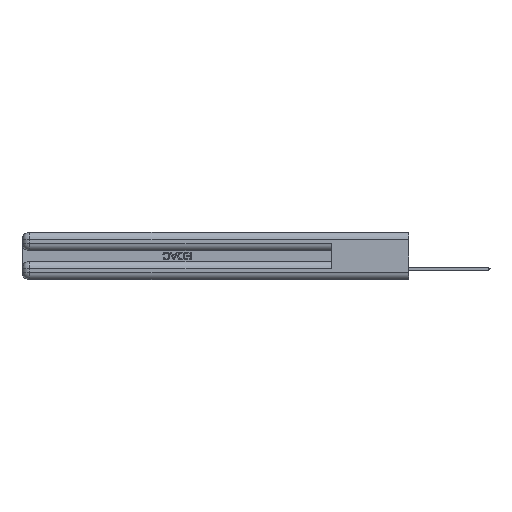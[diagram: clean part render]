
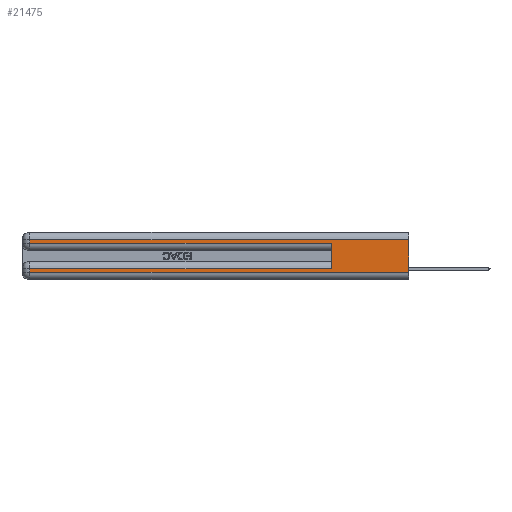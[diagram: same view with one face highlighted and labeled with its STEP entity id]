
A CAD part, left-side view. The second image highlights one B-rep face of the part: STEP entity #21475.
In plain terms, the highlighted planar face has unit normal (-1, 0, 0).
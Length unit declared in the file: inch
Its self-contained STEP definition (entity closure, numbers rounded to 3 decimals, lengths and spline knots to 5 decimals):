
#2013 = VECTOR ( 'NONE', #28800, 39.37008 ) ;
#2244 = DIRECTION ( 'NONE',  ( 0., 0., -1. ) ) ;
#2348 = AXIS2_PLACEMENT_3D ( 'NONE', #2949, #3108, #23574 ) ;
#2818 = DIRECTION ( 'NONE',  ( 0., -1., 0. ) ) ;
#2949 = CARTESIAN_POINT ( 'NONE',  ( 0., 0., 0.37 ) ) ;
#3108 = DIRECTION ( 'NONE',  ( 1., 0., 0. ) ) ;
#3321 = EDGE_CURVE ( 'NONE', #38201, #8779, #11800, .T. ) ;
#3436 = LINE ( 'NONE', #38410, #30275 ) ;
#3728 = LINE ( 'NONE', #9782, #32764 ) ;
#5554 = VERTEX_POINT ( 'NONE', #9610 ) ;
#7257 = EDGE_CURVE ( 'NONE', #16103, #8779, #3728, .T. ) ;
#7358 = CARTESIAN_POINT ( 'NONE',  ( 0., 0., 0.31 ) ) ;
#8779 = VERTEX_POINT ( 'NONE', #22190 ) ;
#9610 = CARTESIAN_POINT ( 'NONE',  ( 0., 2.94, 0.085 ) ) ;
#9782 = CARTESIAN_POINT ( 'NONE',  ( 0., 0., 0.37 ) ) ;
#10537 = ORIENTED_EDGE ( 'NONE', *, *, #3321, .T. ) ;
#11504 = DIRECTION ( 'NONE',  ( 0., 0., -1. ) ) ;
#11552 = LINE ( 'NONE', #16297, #13139 ) ;
#11800 = LINE ( 'NONE', #13578, #14001 ) ;
#12268 = EDGE_CURVE ( 'NONE', #43119, #5554, #11552, .T. ) ;
#12500 = EDGE_LOOP ( 'NONE', ( #44395, #36918, #36871, #23551, #28373, #17682, #26992, #10537 ) ) ;
#13139 = VECTOR ( 'NONE', #19790, 39.37008 ) ;
#13212 = CARTESIAN_POINT ( 'NONE',  ( 0., 0.6, 0.285 ) ) ;
#13380 = VECTOR ( 'NONE', #19745, 39.37008 ) ;
#13578 = CARTESIAN_POINT ( 'NONE',  ( 0., 0., 0.06 ) ) ;
#13644 = CARTESIAN_POINT ( 'NONE',  ( 0., 0.6, 0.085 ) ) ;
#14001 = VECTOR ( 'NONE', #2818, 39.37008 ) ;
#16103 = VERTEX_POINT ( 'NONE', #7358 ) ;
#16235 = EDGE_CURVE ( 'NONE', #45149, #21847, #43623, .T. ) ;
#16279 = VECTOR ( 'NONE', #11504, 39.37008 ) ;
#16297 = CARTESIAN_POINT ( 'NONE',  ( 0., 0., 0.085 ) ) ;
#17682 = ORIENTED_EDGE ( 'NONE', *, *, #12268, .T. ) ;
#17805 = DIRECTION ( 'NONE',  ( 0., 0., 1. ) ) ;
#18359 = CARTESIAN_POINT ( 'NONE',  ( 0., 2.94, 0.285 ) ) ;
#19745 = DIRECTION ( 'NONE',  ( 0., -1., 0. ) ) ;
#19790 = DIRECTION ( 'NONE',  ( 0., 1., 0. ) ) ;
#20095 = LINE ( 'NONE', #41680, #2013 ) ;
#20355 = CARTESIAN_POINT ( 'NONE',  ( 0., 2.94, 0.31 ) ) ;
#21475 = ADVANCED_FACE ( 'NONE', ( #26162 ), #27422, .F. ) ;
#21504 = VERTEX_POINT ( 'NONE', #13212 ) ;
#21847 = VERTEX_POINT ( 'NONE', #18359 ) ;
#22190 = CARTESIAN_POINT ( 'NONE',  ( 0., 0., 0.06 ) ) ;
#23551 = ORIENTED_EDGE ( 'NONE', *, *, #32117, .T. ) ;
#23574 = DIRECTION ( 'NONE',  ( 0., 0., -1. ) ) ;
#23740 = LINE ( 'NONE', #43186, #13380 ) ;
#25168 = EDGE_CURVE ( 'NONE', #16103, #45149, #3436, .T. ) ;
#25958 = EDGE_CURVE ( 'NONE', #43119, #21504, #35446, .T. ) ;
#26162 = FACE_OUTER_BOUND ( 'NONE', #12500, .T. ) ;
#26992 = ORIENTED_EDGE ( 'NONE', *, *, #29769, .T. ) ;
#27422 = PLANE ( 'NONE',  #2348 ) ;
#28262 = VECTOR ( 'NONE', #17805, 39.37008 ) ;
#28373 = ORIENTED_EDGE ( 'NONE', *, *, #25958, .F. ) ;
#28800 = DIRECTION ( 'NONE',  ( 0., 0., -1. ) ) ;
#29769 = EDGE_CURVE ( 'NONE', #5554, #38201, #20095, .T. ) ;
#30275 = VECTOR ( 'NONE', #45324, 39.37008 ) ;
#32117 = EDGE_CURVE ( 'NONE', #21847, #21504, #23740, .T. ) ;
#32764 = VECTOR ( 'NONE', #2244, 39.37008 ) ;
#35446 = LINE ( 'NONE', #38787, #28262 ) ;
#36871 = ORIENTED_EDGE ( 'NONE', *, *, #16235, .T. ) ;
#36918 = ORIENTED_EDGE ( 'NONE', *, *, #25168, .T. ) ;
#36971 = CARTESIAN_POINT ( 'NONE',  ( 0., 2.94, 0.06 ) ) ;
#38201 = VERTEX_POINT ( 'NONE', #36971 ) ;
#38410 = CARTESIAN_POINT ( 'NONE',  ( 0., 0., 0.31 ) ) ;
#38787 = CARTESIAN_POINT ( 'NONE',  ( 0., 0.6, 0.145 ) ) ;
#39370 = CARTESIAN_POINT ( 'NONE',  ( 0., 2.94, 0.37 ) ) ;
#41680 = CARTESIAN_POINT ( 'NONE',  ( 0., 2.94, 0.37 ) ) ;
#43119 = VERTEX_POINT ( 'NONE', #13644 ) ;
#43186 = CARTESIAN_POINT ( 'NONE',  ( 0., 0., 0.285 ) ) ;
#43623 = LINE ( 'NONE', #39370, #16279 ) ;
#44395 = ORIENTED_EDGE ( 'NONE', *, *, #7257, .F. ) ;
#45149 = VERTEX_POINT ( 'NONE', #20355 ) ;
#45324 = DIRECTION ( 'NONE',  ( 0., 1., 0. ) ) ;
